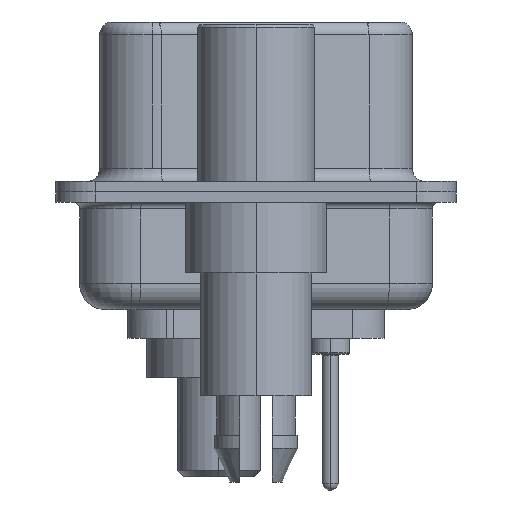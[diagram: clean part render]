
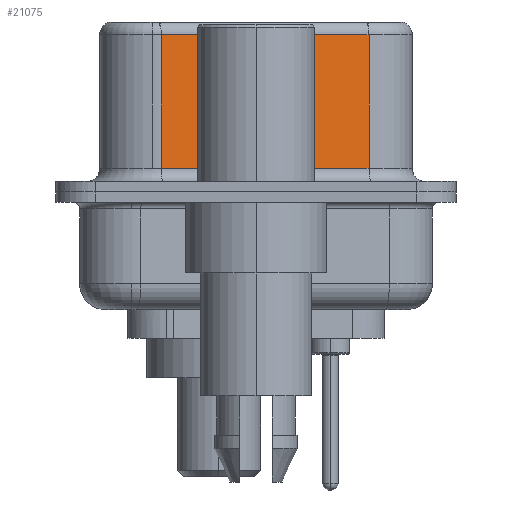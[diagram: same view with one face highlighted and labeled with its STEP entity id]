
A CAD part, left-side view. The second image highlights one B-rep face of the part: STEP entity #21075.
In plain terms, the highlighted planar face has unit normal (-0.985, -0.174, 0).
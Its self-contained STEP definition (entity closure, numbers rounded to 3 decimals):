
#1618 = VECTOR ( 'NONE', #18793, 1000. ) ;
#3057 = LINE ( 'NONE', #6471, #19686 ) ;
#3198 = EDGE_CURVE ( 'NONE', #8720, #21339, #5581, .T. ) ;
#3502 = VERTEX_POINT ( 'NONE', #10291 ) ;
#4223 = ORIENTED_EDGE ( 'NONE', *, *, #10310, .T. ) ;
#4684 = CARTESIAN_POINT ( 'NONE',  ( 5.132, -4.322, 6.02 ) ) ;
#5581 = LINE ( 'NONE', #20623, #1618 ) ;
#5700 = EDGE_LOOP ( 'NONE', ( #16037, #14079, #4223, #18215 ) ) ;
#6266 = DIRECTION ( 'NONE',  ( -0.174, 0.985, 0. ) ) ;
#6361 = LINE ( 'NONE', #7499, #14639 ) ;
#6408 = DIRECTION ( 'NONE',  ( 0., 0., -1. ) ) ;
#6471 = CARTESIAN_POINT ( 'NONE',  ( 3.73, 3.628, 6.52 ) ) ;
#6617 = FACE_OUTER_BOUND ( 'NONE', #5700, .T. ) ;
#6931 = CARTESIAN_POINT ( 'NONE',  ( 5.132, -4.322, 0.9 ) ) ;
#7499 = CARTESIAN_POINT ( 'NONE',  ( 5.132, -4.322, 0.9 ) ) ;
#7815 = VERTEX_POINT ( 'NONE', #9147 ) ;
#8609 = VECTOR ( 'NONE', #17969, 1000. ) ;
#8720 = VERTEX_POINT ( 'NONE', #9288 ) ;
#8855 = EDGE_CURVE ( 'NONE', #8720, #3502, #18430, .T. ) ;
#9147 = CARTESIAN_POINT ( 'NONE',  ( 3.73, 3.628, 0.9 ) ) ;
#9288 = CARTESIAN_POINT ( 'NONE',  ( 5.132, -4.322, 6.02 ) ) ;
#10291 = CARTESIAN_POINT ( 'NONE',  ( 3.73, 3.628, 6.02 ) ) ;
#10310 = EDGE_CURVE ( 'NONE', #3502, #7815, #3057, .T. ) ;
#11209 = CARTESIAN_POINT ( 'NONE',  ( 5.132, -4.322, 6.52 ) ) ;
#13243 = EDGE_CURVE ( 'NONE', #7815, #21339, #6361, .T. ) ;
#14079 = ORIENTED_EDGE ( 'NONE', *, *, #8855, .T. ) ;
#14512 = PLANE ( 'NONE',  #16666 ) ;
#14639 = VECTOR ( 'NONE', #20745, 1000. ) ;
#16037 = ORIENTED_EDGE ( 'NONE', *, *, #3198, .F. ) ;
#16190 = DIRECTION ( 'NONE',  ( 0.985, 0.174, 0. ) ) ;
#16666 = AXIS2_PLACEMENT_3D ( 'NONE', #11209, #16190, #6266 ) ;
#17969 = DIRECTION ( 'NONE',  ( -0.174, 0.985, 0. ) ) ;
#18215 = ORIENTED_EDGE ( 'NONE', *, *, #13243, .T. ) ;
#18430 = LINE ( 'NONE', #4684, #8609 ) ;
#18793 = DIRECTION ( 'NONE',  ( 0., 0., -1. ) ) ;
#19686 = VECTOR ( 'NONE', #6408, 1000. ) ;
#20623 = CARTESIAN_POINT ( 'NONE',  ( 5.132, -4.322, 6.52 ) ) ;
#20745 = DIRECTION ( 'NONE',  ( 0.174, -0.985, 0. ) ) ;
#21075 = ADVANCED_FACE ( 'NONE', ( #6617 ), #14512, .F. ) ;
#21339 = VERTEX_POINT ( 'NONE', #6931 ) ;
